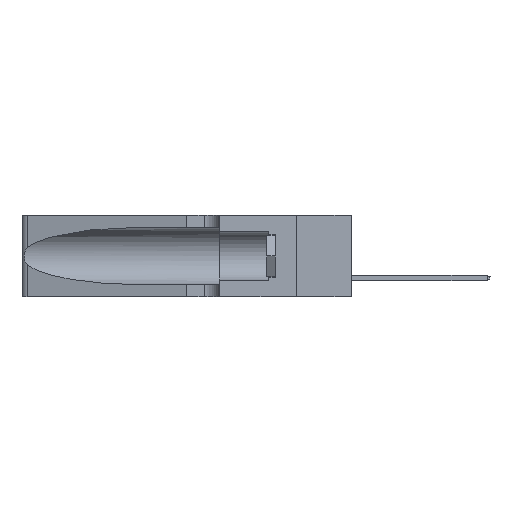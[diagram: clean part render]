
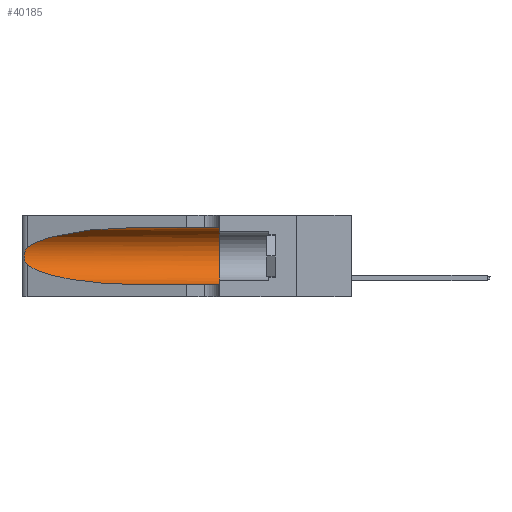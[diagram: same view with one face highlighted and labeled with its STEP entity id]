
A CAD part, left-side view. The second image highlights one B-rep face of the part: STEP entity #40185.
In plain terms, the highlighted cylindrical face has radius 3.308 mm (diameter 6.617 mm), a partial arc.
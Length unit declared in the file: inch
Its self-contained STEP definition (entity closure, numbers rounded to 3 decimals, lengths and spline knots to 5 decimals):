
#1302 = CARTESIAN_POINT ( 'NONE',  ( 0.1305, 1.61858, 0.05475 ) ) ;
#1746 = EDGE_CURVE ( 'NONE', #44786, #18479, #18893, .T. ) ;
#3731 = CARTESIAN_POINT ( 'NONE',  ( 0.26075, 1.23896, 0.178 ) ) ;
#3894 = CARTESIAN_POINT ( 'NONE',  ( 0.1305, 1.61858, 0.185 ) ) ;
#4380 = DIRECTION ( 'NONE',  ( 0., 0., -1. ) ) ;
#5130 = VECTOR ( 'NONE', #33108, 39.37008 ) ;
#6843 = ORIENTED_EDGE ( 'NONE', *, *, #40141, .T. ) ;
#7663 = CARTESIAN_POINT ( 'NONE',  ( 0.25639, 1.23184, 0.21858 ) ) ;
#7986 = CARTESIAN_POINT ( 'NONE',  ( 0.25856, 1.23593, 0.16098 ) ) ;
#8309 = CARTESIAN_POINT ( 'NONE',  ( 0.25639, 1.23186, 0.15144 ) ) ;
#8643 = FACE_OUTER_BOUND ( 'NONE', #44663, .T. ) ;
#11639 = CARTESIAN_POINT ( 'NONE',  ( 0.25555, 1.22994, 0.2215 ) ) ;
#14082 = DIRECTION ( 'NONE',  ( 0., 0., 1. ) ) ;
#15075 = CARTESIAN_POINT ( 'NONE',  ( 0.1305, 0.72297, 0.31525 ) ) ;
#15104 = EDGE_CURVE ( 'NONE', #39251, #34361, #47035, .T. ) ;
#15310 = CARTESIAN_POINT ( 'NONE',  ( 0.2373, 1.15595, 0.08982 ) ) ;
#15334 = CARTESIAN_POINT ( 'NONE',  ( 0.26018, 1.23835, 0.19895 ) ) ;
#15740 = AXIS2_PLACEMENT_3D ( 'NONE', #3894, #23921, #4380 ) ;
#18479 = VERTEX_POINT ( 'NONE', #26438 ) ;
#18548 = ORIENTED_EDGE ( 'NONE', *, *, #36098, .T. ) ;
#18680 = ORIENTED_EDGE ( 'NONE', *, *, #15104, .T. ) ;
#18893 = LINE ( 'NONE', #26147, #36681 ) ;
#20577 = VERTEX_POINT ( 'NONE', #22758 ) ;
#22355 = CYLINDRICAL_SURFACE ( 'NONE', #15740, 0.13025 ) ;
#22758 = CARTESIAN_POINT ( 'NONE',  ( 0.25487, 1.22718, 0.22369 ) ) ;
#23558 = CARTESIAN_POINT ( 'NONE',  ( 0.1305, 0.72297, 0.05475 ) ) ;
#23921 = DIRECTION ( 'NONE',  ( 0., -1., 0. ) ) ;
#24179 = CARTESIAN_POINT ( 'NONE',  ( 0.18966, 0.96281, 0.31525 ) ) ;
#25470 =( BOUNDED_CURVE ( )  B_SPLINE_CURVE ( 3, ( #46577, #15310, #34604, #23558 ),
 .UNSPECIFIED., .F., .F. ) 
 B_SPLINE_CURVE_WITH_KNOTS ( ( 4, 4 ),
 ( 3.44316, 4.71239 ),
 .UNSPECIFIED. ) 
 CURVE ( )  GEOMETRIC_REPRESENTATION_ITEM ( )  RATIONAL_B_SPLINE_CURVE ( ( 1., 0.87, 0.87, 1. ) ) 
 REPRESENTATION_ITEM ( '' )  );
#26147 = CARTESIAN_POINT ( 'NONE',  ( 0.1305, 1.61858, 0.31525 ) ) ;
#26438 = CARTESIAN_POINT ( 'NONE',  ( 0.1305, 0.35, 0.31525 ) ) ;
#27387 = CARTESIAN_POINT ( 'NONE',  ( 0.25487, 1.22718, 0.22369 ) ) ;
#29941 = CARTESIAN_POINT ( 'NONE',  ( 0.25487, 1.22718, 0.14631 ) ) ;
#29990 = DIRECTION ( 'NONE',  ( 0., 1., 0. ) ) ;
#33108 = DIRECTION ( 'NONE',  ( 0., -1., 0. ) ) ;
#34361 = VERTEX_POINT ( 'NONE', #45223 ) ;
#34604 = CARTESIAN_POINT ( 'NONE',  ( 0.18966, 0.96281, 0.05475 ) ) ;
#34669 = B_SPLINE_CURVE_WITH_KNOTS ( 'NONE', 3,
 ( #27387, #11639, #7663, #50592, #38874, #15334, #42829, #3731, #35766, #7986, #47263, #8309, #35614, #43811 ),
 .UNSPECIFIED., .F., .F.,
 ( 4, 2, 2, 2, 2, 2, 4 ),
 ( 0., 0.00027, 0.00053, 0.00107, 0.0016, 0.00187, 0.00214 ),
 .UNSPECIFIED. ) ;
#35532 = ORIENTED_EDGE ( 'NONE', *, *, #41487, .T. ) ;
#35614 = CARTESIAN_POINT ( 'NONE',  ( 0.25555, 1.22993, 0.14849 ) ) ;
#35766 = CARTESIAN_POINT ( 'NONE',  ( 0.26017, 1.23833, 0.17102 ) ) ;
#36098 = EDGE_CURVE ( 'NONE', #44786, #20577, #50721, .T. ) ;
#36681 = VECTOR ( 'NONE', #47761, 39.37008 ) ;
#38439 = ORIENTED_EDGE ( 'NONE', *, *, #41252, .F. ) ;
#38874 = CARTESIAN_POINT ( 'NONE',  ( 0.25854, 1.2359, 0.20912 ) ) ;
#39251 = VERTEX_POINT ( 'NONE', #47268 ) ;
#39293 = VERTEX_POINT ( 'NONE', #29941 ) ;
#39453 = CARTESIAN_POINT ( 'NONE',  ( 0.25487, 1.22718, 0.22369 ) ) ;
#39777 = CARTESIAN_POINT ( 'NONE',  ( 0.2373, 1.15595, 0.28018 ) ) ;
#40141 = EDGE_CURVE ( 'NONE', #20577, #39293, #34669, .T. ) ;
#40185 = ADVANCED_FACE ( 'NONE', ( #8643 ), #22355, .F. ) ;
#41252 = EDGE_CURVE ( 'NONE', #18479, #34361, #41878, .T. ) ;
#41487 = EDGE_CURVE ( 'NONE', #39293, #39251, #25470, .T. ) ;
#41878 = CIRCLE ( 'NONE', #43727, 0.13025 ) ;
#42829 = CARTESIAN_POINT ( 'NONE',  ( 0.26075, 1.23896, 0.19203 ) ) ;
#43727 = AXIS2_PLACEMENT_3D ( 'NONE', #45898, #29990, #14082 ) ;
#43811 = CARTESIAN_POINT ( 'NONE',  ( 0.25487, 1.22718, 0.14631 ) ) ;
#44663 = EDGE_LOOP ( 'NONE', ( #18548, #6843, #35532, #18680, #38439, #46223 ) ) ;
#44786 = VERTEX_POINT ( 'NONE', #48000 ) ;
#45223 = CARTESIAN_POINT ( 'NONE',  ( 0.1305, 0.35, 0.05475 ) ) ;
#45898 = CARTESIAN_POINT ( 'NONE',  ( 0.1305, 0.35, 0.185 ) ) ;
#46223 = ORIENTED_EDGE ( 'NONE', *, *, #1746, .F. ) ;
#46577 = CARTESIAN_POINT ( 'NONE',  ( 0.25487, 1.22718, 0.14631 ) ) ;
#47035 = LINE ( 'NONE', #1302, #5130 ) ;
#47263 = CARTESIAN_POINT ( 'NONE',  ( 0.25789, 1.23486, 0.15765 ) ) ;
#47268 = CARTESIAN_POINT ( 'NONE',  ( 0.1305, 0.72297, 0.05475 ) ) ;
#47761 = DIRECTION ( 'NONE',  ( 0., -1., 0. ) ) ;
#48000 = CARTESIAN_POINT ( 'NONE',  ( 0.1305, 0.72297, 0.31525 ) ) ;
#50592 = CARTESIAN_POINT ( 'NONE',  ( 0.25787, 1.23484, 0.2124 ) ) ;
#50721 =( BOUNDED_CURVE ( )  B_SPLINE_CURVE ( 3, ( #15075, #24179, #39777, #39453 ),
 .UNSPECIFIED., .F., .F. ) 
 B_SPLINE_CURVE_WITH_KNOTS ( ( 4, 4 ),
 ( 1.5708, 2.84003 ),
 .UNSPECIFIED. ) 
 CURVE ( )  GEOMETRIC_REPRESENTATION_ITEM ( )  RATIONAL_B_SPLINE_CURVE ( ( 1., 0.87, 0.87, 1. ) ) 
 REPRESENTATION_ITEM ( '' )  );
